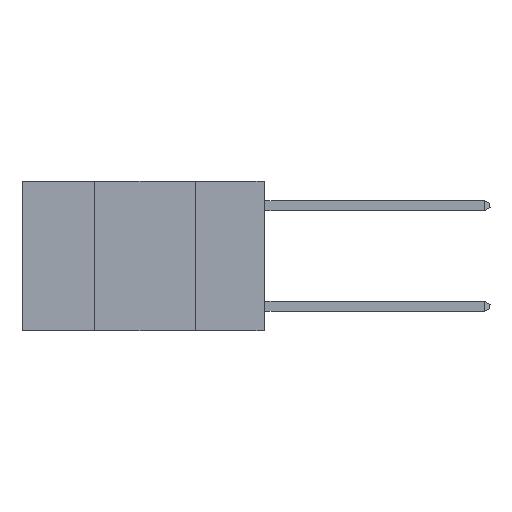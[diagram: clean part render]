
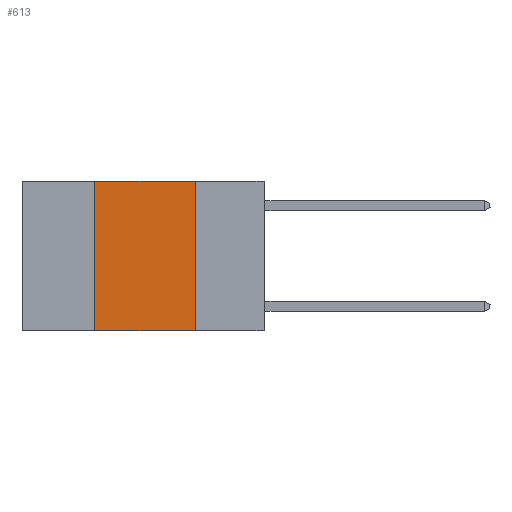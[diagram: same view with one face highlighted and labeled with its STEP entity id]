
A CAD part, left-side view. The second image highlights one B-rep face of the part: STEP entity #613.
In plain terms, the highlighted planar face has unit normal (-1, 0, 0).
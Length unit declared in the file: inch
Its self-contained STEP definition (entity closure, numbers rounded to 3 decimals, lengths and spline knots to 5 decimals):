
#91 = CARTESIAN_POINT ( 'NONE',  ( 0., 0.17, 0. ) ) ;
#273 = DIRECTION ( 'NONE',  ( 0., 0., 1. ) ) ;
#429 = FACE_OUTER_BOUND ( 'NONE', #14420, .T. ) ;
#613 = ADVANCED_FACE ( 'NONE', ( #429 ), #10739, .F. ) ;
#829 = DIRECTION ( 'NONE',  ( 0., -1., 0. ) ) ;
#984 = EDGE_CURVE ( 'NONE', #3751, #13642, #14204, .T. ) ;
#987 = EDGE_CURVE ( 'NONE', #3751, #11839, #11192, .T. ) ;
#1275 = CARTESIAN_POINT ( 'NONE',  ( 0., 0.6, 0. ) ) ;
#2194 = VECTOR ( 'NONE', #829, 39.37008 ) ;
#2590 = LINE ( 'NONE', #3315, #2194 ) ;
#3315 = CARTESIAN_POINT ( 'NONE',  ( 0., 0.6, 0. ) ) ;
#3751 = VERTEX_POINT ( 'NONE', #11358 ) ;
#4170 = ORIENTED_EDGE ( 'NONE', *, *, #7374, .F. ) ;
#5093 = DIRECTION ( 'NONE',  ( 1., 0., 0. ) ) ;
#5242 = CARTESIAN_POINT ( 'NONE',  ( 0., 0.42, 0. ) ) ;
#5476 = VECTOR ( 'NONE', #11001, 39.37008 ) ;
#6127 = DIRECTION ( 'NONE',  ( 0., 0., -1. ) ) ;
#7374 = EDGE_CURVE ( 'NONE', #11839, #10622, #2590, .T. ) ;
#8140 = VECTOR ( 'NONE', #10647, 39.37008 ) ;
#8865 = VECTOR ( 'NONE', #273, 39.37008 ) ;
#8901 = CARTESIAN_POINT ( 'NONE',  ( 0., 0.6, -0.37 ) ) ;
#8908 = LINE ( 'NONE', #9841, #5476 ) ;
#9409 = CARTESIAN_POINT ( 'NONE',  ( 0., 0.17, -0.37 ) ) ;
#9589 = ORIENTED_EDGE ( 'NONE', *, *, #11628, .F. ) ;
#9841 = CARTESIAN_POINT ( 'NONE',  ( 0., 0.17, 0. ) ) ;
#10429 = CARTESIAN_POINT ( 'NONE',  ( 0., 0.42, 0. ) ) ;
#10622 = VERTEX_POINT ( 'NONE', #91 ) ;
#10647 = DIRECTION ( 'NONE',  ( 0., -1., 0. ) ) ;
#10696 = AXIS2_PLACEMENT_3D ( 'NONE', #1275, #5093, #6127 ) ;
#10739 = PLANE ( 'NONE',  #10696 ) ;
#11001 = DIRECTION ( 'NONE',  ( 0., 0., -1. ) ) ;
#11192 = LINE ( 'NONE', #5242, #8865 ) ;
#11358 = CARTESIAN_POINT ( 'NONE',  ( 0., 0.42, -0.37 ) ) ;
#11628 = EDGE_CURVE ( 'NONE', #10622, #13642, #8908, .T. ) ;
#11839 = VERTEX_POINT ( 'NONE', #10429 ) ;
#13001 = ORIENTED_EDGE ( 'NONE', *, *, #987, .F. ) ;
#13642 = VERTEX_POINT ( 'NONE', #9409 ) ;
#13689 = ORIENTED_EDGE ( 'NONE', *, *, #984, .T. ) ;
#14204 = LINE ( 'NONE', #8901, #8140 ) ;
#14420 = EDGE_LOOP ( 'NONE', ( #9589, #4170, #13001, #13689 ) ) ;
